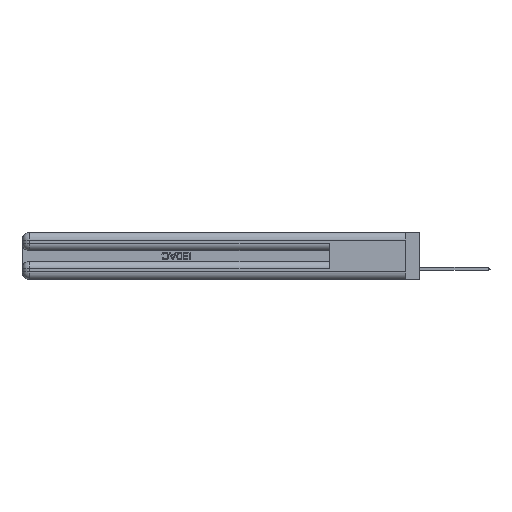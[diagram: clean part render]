
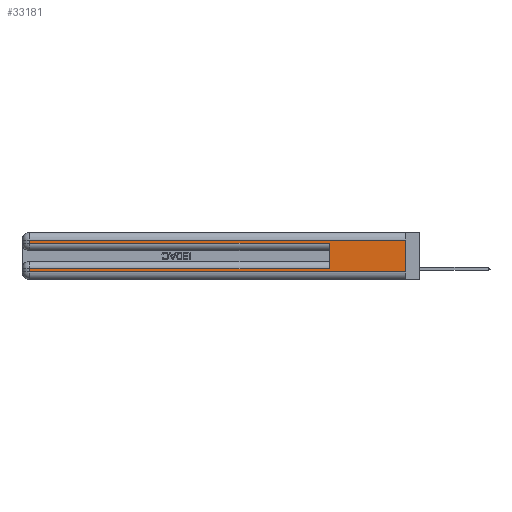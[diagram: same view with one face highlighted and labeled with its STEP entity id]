
A CAD part, left-side view. The second image highlights one B-rep face of the part: STEP entity #33181.
In plain terms, the highlighted planar face has unit normal (-1, 0, 0).
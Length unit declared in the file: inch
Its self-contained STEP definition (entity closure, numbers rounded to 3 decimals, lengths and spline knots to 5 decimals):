
#618 = CARTESIAN_POINT ( 'NONE',  ( 0., 2.94, 0.37 ) ) ;
#1843 = DIRECTION ( 'NONE',  ( 0., 0., -1. ) ) ;
#2143 = DIRECTION ( 'NONE',  ( 0., 1., 0. ) ) ;
#2927 = EDGE_CURVE ( 'NONE', #45833, #31953, #4575, .T. ) ;
#4575 = LINE ( 'NONE', #6221, #47728 ) ;
#4925 = ORIENTED_EDGE ( 'NONE', *, *, #34184, .T. ) ;
#6221 = CARTESIAN_POINT ( 'NONE',  ( 0., 0.6, 0.145 ) ) ;
#6380 = DIRECTION ( 'NONE',  ( 0., 1., 0. ) ) ;
#6620 = CARTESIAN_POINT ( 'NONE',  ( 0., 0., 0.37 ) ) ;
#6711 = ORIENTED_EDGE ( 'NONE', *, *, #51460, .T. ) ;
#8088 = CARTESIAN_POINT ( 'NONE',  ( 0., 0., 0.37 ) ) ;
#8172 = PLANE ( 'NONE',  #21727 ) ;
#8739 = ORIENTED_EDGE ( 'NONE', *, *, #53969, .T. ) ;
#9581 = VECTOR ( 'NONE', #27608, 39.37008 ) ;
#9876 = LINE ( 'NONE', #618, #29050 ) ;
#10859 = CARTESIAN_POINT ( 'NONE',  ( 0., 2.94, 0.085 ) ) ;
#11005 = LINE ( 'NONE', #52645, #9581 ) ;
#12030 = CARTESIAN_POINT ( 'NONE',  ( 0., 0., 0.06 ) ) ;
#13365 = VERTEX_POINT ( 'NONE', #17446 ) ;
#13822 = EDGE_CURVE ( 'NONE', #28021, #31953, #50462, .T. ) ;
#14748 = CARTESIAN_POINT ( 'NONE',  ( 0., 2.94, 0.37 ) ) ;
#15425 = VECTOR ( 'NONE', #42234, 39.37008 ) ;
#17446 = CARTESIAN_POINT ( 'NONE',  ( 0., 0., 0.31 ) ) ;
#17760 = CARTESIAN_POINT ( 'NONE',  ( 0., 2.94, 0.06 ) ) ;
#19361 = CARTESIAN_POINT ( 'NONE',  ( 0., 2.94, 0.31 ) ) ;
#21263 = EDGE_LOOP ( 'NONE', ( #22268, #4925, #6711, #40946, #38951, #8739, #26975, #33154 ) ) ;
#21727 = AXIS2_PLACEMENT_3D ( 'NONE', #6620, #51898, #23068 ) ;
#22268 = ORIENTED_EDGE ( 'NONE', *, *, #42354, .F. ) ;
#22453 = LINE ( 'NONE', #14748, #51908 ) ;
#22462 = LINE ( 'NONE', #8088, #15425 ) ;
#23068 = DIRECTION ( 'NONE',  ( 0., 0., -1. ) ) ;
#23298 = VERTEX_POINT ( 'NONE', #17760 ) ;
#24420 = VECTOR ( 'NONE', #6380, 39.37008 ) ;
#26883 = VECTOR ( 'NONE', #2143, 39.37008 ) ;
#26975 = ORIENTED_EDGE ( 'NONE', *, *, #53709, .T. ) ;
#27199 = VERTEX_POINT ( 'NONE', #19361 ) ;
#27368 = CARTESIAN_POINT ( 'NONE',  ( 0., 0.6, 0.285 ) ) ;
#27473 = CARTESIAN_POINT ( 'NONE',  ( 0., 0., 0.085 ) ) ;
#27579 = VECTOR ( 'NONE', #30270, 39.37008 ) ;
#27608 = DIRECTION ( 'NONE',  ( 0., -1., 0. ) ) ;
#28021 = VERTEX_POINT ( 'NONE', #31412 ) ;
#29050 = VECTOR ( 'NONE', #34412, 39.37008 ) ;
#30270 = DIRECTION ( 'NONE',  ( 0., -1., 0. ) ) ;
#30284 = FACE_OUTER_BOUND ( 'NONE', #21263, .T. ) ;
#31412 = CARTESIAN_POINT ( 'NONE',  ( 0., 2.94, 0.285 ) ) ;
#31953 = VERTEX_POINT ( 'NONE', #27368 ) ;
#33154 = ORIENTED_EDGE ( 'NONE', *, *, #38688, .T. ) ;
#33181 = ADVANCED_FACE ( 'NONE', ( #30284 ), #8172, .F. ) ;
#33610 = CARTESIAN_POINT ( 'NONE',  ( 0., 0., 0.31 ) ) ;
#33800 = VERTEX_POINT ( 'NONE', #10859 ) ;
#34184 = EDGE_CURVE ( 'NONE', #13365, #27199, #50466, .T. ) ;
#34412 = DIRECTION ( 'NONE',  ( 0., 0., -1. ) ) ;
#38688 = EDGE_CURVE ( 'NONE', #23298, #43057, #11005, .T. ) ;
#38951 = ORIENTED_EDGE ( 'NONE', *, *, #2927, .F. ) ;
#40946 = ORIENTED_EDGE ( 'NONE', *, *, #13822, .T. ) ;
#42234 = DIRECTION ( 'NONE',  ( 0., 0., -1. ) ) ;
#42354 = EDGE_CURVE ( 'NONE', #13365, #43057, #22462, .T. ) ;
#43057 = VERTEX_POINT ( 'NONE', #12030 ) ;
#44135 = DIRECTION ( 'NONE',  ( 0., 0., 1. ) ) ;
#45366 = LINE ( 'NONE', #27473, #24420 ) ;
#45833 = VERTEX_POINT ( 'NONE', #50194 ) ;
#47728 = VECTOR ( 'NONE', #44135, 39.37008 ) ;
#50194 = CARTESIAN_POINT ( 'NONE',  ( 0., 0.6, 0.085 ) ) ;
#50462 = LINE ( 'NONE', #54040, #27579 ) ;
#50466 = LINE ( 'NONE', #33610, #26883 ) ;
#51460 = EDGE_CURVE ( 'NONE', #27199, #28021, #22453, .T. ) ;
#51898 = DIRECTION ( 'NONE',  ( 1., 0., 0. ) ) ;
#51908 = VECTOR ( 'NONE', #1843, 39.37008 ) ;
#52645 = CARTESIAN_POINT ( 'NONE',  ( 0., 0., 0.06 ) ) ;
#53709 = EDGE_CURVE ( 'NONE', #33800, #23298, #9876, .T. ) ;
#53969 = EDGE_CURVE ( 'NONE', #45833, #33800, #45366, .T. ) ;
#54040 = CARTESIAN_POINT ( 'NONE',  ( 0., 0., 0.285 ) ) ;
